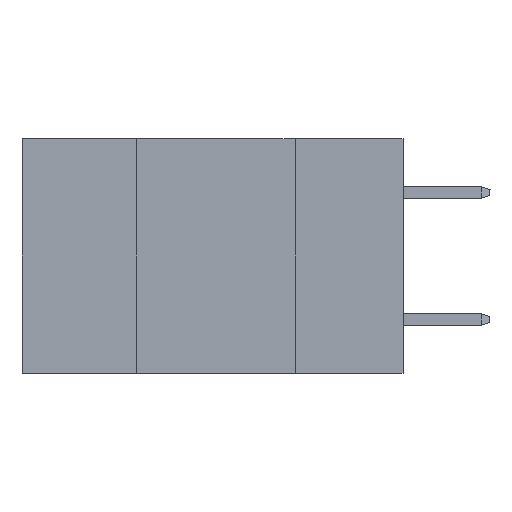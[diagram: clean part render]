
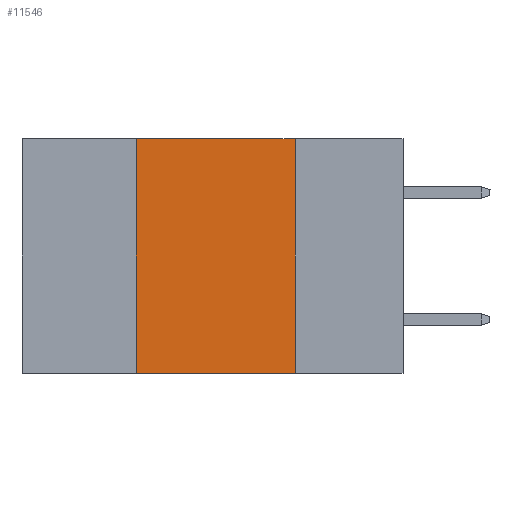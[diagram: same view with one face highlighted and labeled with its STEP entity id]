
A CAD part, left-side view. The second image highlights one B-rep face of the part: STEP entity #11546.
In plain terms, the highlighted planar face has unit normal (-1, 0, 0).
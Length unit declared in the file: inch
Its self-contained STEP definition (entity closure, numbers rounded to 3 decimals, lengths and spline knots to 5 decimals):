
#889 = LINE ( 'NONE', #10369, #2656 ) ;
#1772 = LINE ( 'NONE', #9785, #4907 ) ;
#2063 = VERTEX_POINT ( 'NONE', #16571 ) ;
#2508 = VECTOR ( 'NONE', #5363, 39.37008 ) ;
#2656 = VECTOR ( 'NONE', #8890, 39.37008 ) ;
#3353 = ORIENTED_EDGE ( 'NONE', *, *, #5854, .F. ) ;
#3815 = AXIS2_PLACEMENT_3D ( 'NONE', #9601, #11279, #11591 ) ;
#4282 = VERTEX_POINT ( 'NONE', #4464 ) ;
#4464 = CARTESIAN_POINT ( 'NONE',  ( 0., 0.17, -0.37 ) ) ;
#4907 = VECTOR ( 'NONE', #14622, 39.37008 ) ;
#5187 = LINE ( 'NONE', #13481, #7149 ) ;
#5363 = DIRECTION ( 'NONE',  ( 0., 0., 1. ) ) ;
#5376 = ORIENTED_EDGE ( 'NONE', *, *, #16171, .T. ) ;
#5854 = EDGE_CURVE ( 'NONE', #7314, #2063, #5187, .T. ) ;
#5964 = ORIENTED_EDGE ( 'NONE', *, *, #14817, .F. ) ;
#7149 = VECTOR ( 'NONE', #11605, 39.37008 ) ;
#7314 = VERTEX_POINT ( 'NONE', #13363 ) ;
#8284 = EDGE_LOOP ( 'NONE', ( #15881, #3353, #5964, #5376 ) ) ;
#8890 = DIRECTION ( 'NONE',  ( 0., 0., -1. ) ) ;
#9601 = CARTESIAN_POINT ( 'NONE',  ( 0., 0.6, 0. ) ) ;
#9785 = CARTESIAN_POINT ( 'NONE',  ( 0., 0.6, -0.37 ) ) ;
#10369 = CARTESIAN_POINT ( 'NONE',  ( 0., 0.17, 0. ) ) ;
#11279 = DIRECTION ( 'NONE',  ( 1., 0., 0. ) ) ;
#11374 = FACE_OUTER_BOUND ( 'NONE', #8284, .T. ) ;
#11546 = ADVANCED_FACE ( 'NONE', ( #11374 ), #14626, .F. ) ;
#11575 = LINE ( 'NONE', #16361, #2508 ) ;
#11591 = DIRECTION ( 'NONE',  ( 0., 0., -1. ) ) ;
#11605 = DIRECTION ( 'NONE',  ( 0., -1., 0. ) ) ;
#13363 = CARTESIAN_POINT ( 'NONE',  ( 0., 0.42, 0. ) ) ;
#13481 = CARTESIAN_POINT ( 'NONE',  ( 0., 0.6, 0. ) ) ;
#14622 = DIRECTION ( 'NONE',  ( 0., -1., 0. ) ) ;
#14626 = PLANE ( 'NONE',  #3815 ) ;
#14817 = EDGE_CURVE ( 'NONE', #19222, #7314, #11575, .T. ) ;
#15881 = ORIENTED_EDGE ( 'NONE', *, *, #19849, .F. ) ;
#16171 = EDGE_CURVE ( 'NONE', #19222, #4282, #1772, .T. ) ;
#16361 = CARTESIAN_POINT ( 'NONE',  ( 0., 0.42, 0. ) ) ;
#16571 = CARTESIAN_POINT ( 'NONE',  ( 0., 0.17, 0. ) ) ;
#19222 = VERTEX_POINT ( 'NONE', #19700 ) ;
#19700 = CARTESIAN_POINT ( 'NONE',  ( 0., 0.42, -0.37 ) ) ;
#19849 = EDGE_CURVE ( 'NONE', #2063, #4282, #889, .T. ) ;
